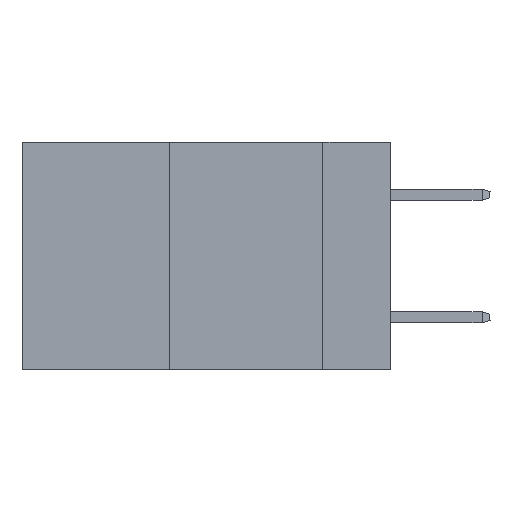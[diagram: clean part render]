
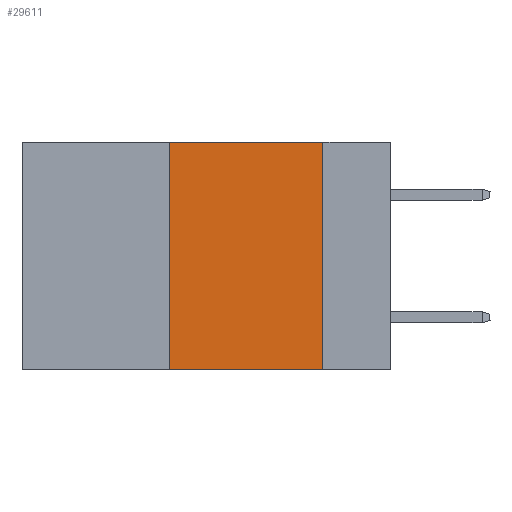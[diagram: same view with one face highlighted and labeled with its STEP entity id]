
A CAD part, left-side view. The second image highlights one B-rep face of the part: STEP entity #29611.
In plain terms, the highlighted planar face has unit normal (-1, 0, 0).
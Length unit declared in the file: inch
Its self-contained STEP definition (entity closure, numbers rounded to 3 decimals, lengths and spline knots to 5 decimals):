
#591 = ORIENTED_EDGE ( 'NONE', *, *, #30400, .F. ) ;
#1346 = DIRECTION ( 'NONE',  ( 0., 0., -1. ) ) ;
#2142 = DIRECTION ( 'NONE',  ( 0., -1., 0. ) ) ;
#2517 = CARTESIAN_POINT ( 'NONE',  ( 0., 0.11, 0. ) ) ;
#4097 = DIRECTION ( 'NONE',  ( 0., 0., 1. ) ) ;
#4629 = EDGE_LOOP ( 'NONE', ( #28567, #591, #26973, #19590 ) ) ;
#6463 = EDGE_CURVE ( 'NONE', #32422, #32357, #30587, .T. ) ;
#8862 = AXIS2_PLACEMENT_3D ( 'NONE', #33268, #17612, #1346 ) ;
#12110 = DIRECTION ( 'NONE',  ( 0., -1., 0. ) ) ;
#12816 = CARTESIAN_POINT ( 'NONE',  ( 0., 0.11, -0.37 ) ) ;
#13471 = CARTESIAN_POINT ( 'NONE',  ( 0., 0.36, -0.37 ) ) ;
#14906 = CARTESIAN_POINT ( 'NONE',  ( 0., 0.36, 0. ) ) ;
#14918 = PLANE ( 'NONE',  #8862 ) ;
#15577 = FACE_OUTER_BOUND ( 'NONE', #4629, .T. ) ;
#15806 = VECTOR ( 'NONE', #4097, 39.37008 ) ;
#16038 = VERTEX_POINT ( 'NONE', #12816 ) ;
#17612 = DIRECTION ( 'NONE',  ( 1., 0., 0. ) ) ;
#19590 = ORIENTED_EDGE ( 'NONE', *, *, #20789, .T. ) ;
#19665 = LINE ( 'NONE', #34025, #24991 ) ;
#20789 = EDGE_CURVE ( 'NONE', #32422, #16038, #34156, .T. ) ;
#22617 = VECTOR ( 'NONE', #25380, 39.37008 ) ;
#22778 = CARTESIAN_POINT ( 'NONE',  ( 0., 0.11, 0. ) ) ;
#23789 = CARTESIAN_POINT ( 'NONE',  ( 0., 0.36, 0. ) ) ;
#24991 = VECTOR ( 'NONE', #2142, 39.37008 ) ;
#25293 = CARTESIAN_POINT ( 'NONE',  ( 0., 0.6, -0.37 ) ) ;
#25380 = DIRECTION ( 'NONE',  ( 0., 0., -1. ) ) ;
#26973 = ORIENTED_EDGE ( 'NONE', *, *, #6463, .F. ) ;
#27219 = VECTOR ( 'NONE', #12110, 39.37008 ) ;
#28567 = ORIENTED_EDGE ( 'NONE', *, *, #29591, .F. ) ;
#29591 = EDGE_CURVE ( 'NONE', #29929, #16038, #30383, .T. ) ;
#29611 = ADVANCED_FACE ( 'NONE', ( #15577 ), #14918, .F. ) ;
#29929 = VERTEX_POINT ( 'NONE', #2517 ) ;
#30383 = LINE ( 'NONE', #22778, #22617 ) ;
#30400 = EDGE_CURVE ( 'NONE', #32357, #29929, #19665, .T. ) ;
#30587 = LINE ( 'NONE', #14906, #15806 ) ;
#32357 = VERTEX_POINT ( 'NONE', #23789 ) ;
#32422 = VERTEX_POINT ( 'NONE', #13471 ) ;
#33268 = CARTESIAN_POINT ( 'NONE',  ( 0., 0.6, 0. ) ) ;
#34025 = CARTESIAN_POINT ( 'NONE',  ( 0., 0.6, 0. ) ) ;
#34156 = LINE ( 'NONE', #25293, #27219 ) ;
